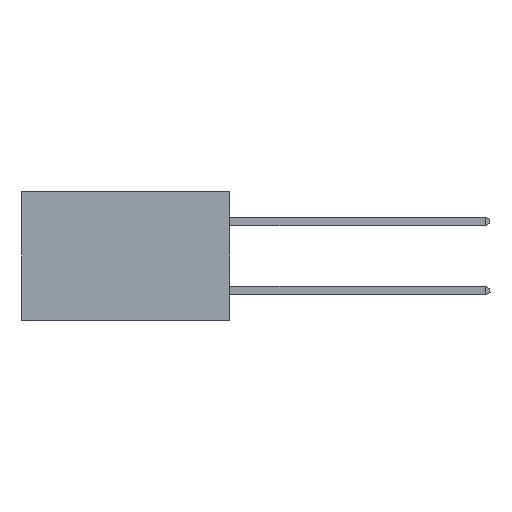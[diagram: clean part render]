
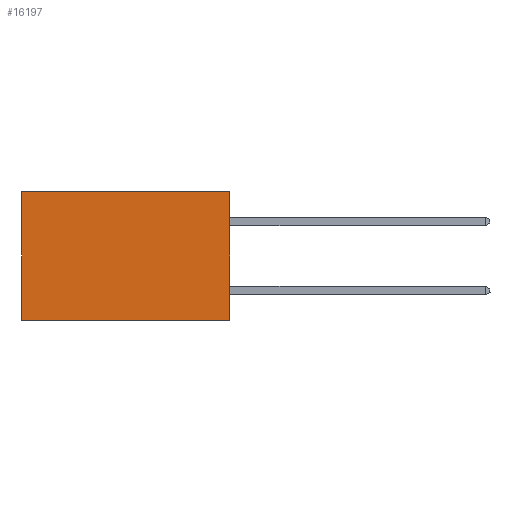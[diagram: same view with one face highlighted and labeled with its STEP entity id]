
A CAD part, left-side view. The second image highlights one B-rep face of the part: STEP entity #16197.
In plain terms, the highlighted planar face has unit normal (-1, 0, 0).
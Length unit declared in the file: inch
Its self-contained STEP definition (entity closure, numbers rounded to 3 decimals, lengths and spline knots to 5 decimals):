
#247 = LINE ( 'NONE', #23679, #13446 ) ;
#1556 = DIRECTION ( 'NONE',  ( 1., 0., 0. ) ) ;
#2401 = CARTESIAN_POINT ( 'NONE',  ( 0.298, 0., -0.37 ) ) ;
#3056 = VECTOR ( 'NONE', #4595, 39.37008 ) ;
#3313 = DIRECTION ( 'NONE',  ( 0., 0., -1. ) ) ;
#3568 = DIRECTION ( 'NONE',  ( 0., 0., -1. ) ) ;
#4595 = DIRECTION ( 'NONE',  ( 0., 1., 0. ) ) ;
#4913 = ORIENTED_EDGE ( 'NONE', *, *, #19018, .T. ) ;
#5184 = EDGE_CURVE ( 'NONE', #18535, #15791, #247, .T. ) ;
#5648 = CARTESIAN_POINT ( 'NONE',  ( 0.298, 0., 0. ) ) ;
#5934 = DIRECTION ( 'NONE',  ( 0., 0., -1. ) ) ;
#6622 = LINE ( 'NONE', #25148, #3056 ) ;
#8032 = VECTOR ( 'NONE', #12536, 39.37008 ) ;
#8531 = FACE_OUTER_BOUND ( 'NONE', #16414, .T. ) ;
#9423 = VECTOR ( 'NONE', #3568, 39.37008 ) ;
#9473 = LINE ( 'NONE', #26234, #8032 ) ;
#12265 = ORIENTED_EDGE ( 'NONE', *, *, #5184, .T. ) ;
#12536 = DIRECTION ( 'NONE',  ( 0., 1., 0. ) ) ;
#13446 = VECTOR ( 'NONE', #3313, 39.37008 ) ;
#14376 = ORIENTED_EDGE ( 'NONE', *, *, #25108, .F. ) ;
#15791 = VERTEX_POINT ( 'NONE', #25142 ) ;
#16197 = ADVANCED_FACE ( 'NONE', ( #8531 ), #17506, .F. ) ;
#16414 = EDGE_LOOP ( 'NONE', ( #12265, #21728, #14376, #4913 ) ) ;
#17309 = CARTESIAN_POINT ( 'NONE',  ( 0.298, 0., 0. ) ) ;
#17506 = PLANE ( 'NONE',  #18164 ) ;
#18164 = AXIS2_PLACEMENT_3D ( 'NONE', #17309, #1556, #5934 ) ;
#18535 = VERTEX_POINT ( 'NONE', #26170 ) ;
#19018 = EDGE_CURVE ( 'NONE', #26198, #18535, #6622, .T. ) ;
#19356 = EDGE_CURVE ( 'NONE', #24922, #15791, #9473, .T. ) ;
#19757 = LINE ( 'NONE', #5648, #9423 ) ;
#20781 = CARTESIAN_POINT ( 'NONE',  ( 0.298, 0., 0. ) ) ;
#21728 = ORIENTED_EDGE ( 'NONE', *, *, #19356, .F. ) ;
#23679 = CARTESIAN_POINT ( 'NONE',  ( 0.298, 0.6, 0. ) ) ;
#24922 = VERTEX_POINT ( 'NONE', #2401 ) ;
#25108 = EDGE_CURVE ( 'NONE', #26198, #24922, #19757, .T. ) ;
#25142 = CARTESIAN_POINT ( 'NONE',  ( 0.298, 0.6, -0.37 ) ) ;
#25148 = CARTESIAN_POINT ( 'NONE',  ( 0.298, 0., 0. ) ) ;
#26170 = CARTESIAN_POINT ( 'NONE',  ( 0.298, 0.6, 0. ) ) ;
#26198 = VERTEX_POINT ( 'NONE', #20781 ) ;
#26234 = CARTESIAN_POINT ( 'NONE',  ( 0.298, 0., -0.37 ) ) ;
